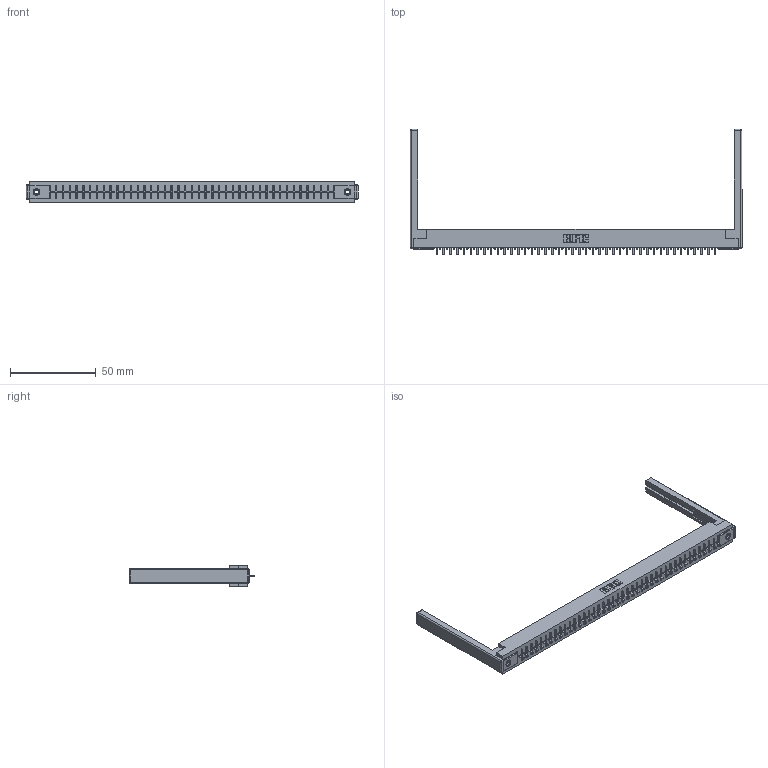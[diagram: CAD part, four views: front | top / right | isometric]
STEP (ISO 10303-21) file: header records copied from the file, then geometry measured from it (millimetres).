
FILE_DESCRIPTION (( 'STEP AP203' ), '1' );
FILE_NAME ('306-042-521-168.STEP', '2019-09-12T00:56:24', ( '' ), ( '' ), 'SwSTEP 2.0', 'SolidWorks 2016', '' );
FILE_SCHEMA (( 'CONFIG_CONTROL_DESIGN' ));
Length unit declared in the file: inch
Products named in the file (5): 345-250-001_345-250-001-102; 306-042-521-168; 307-220-068; 306-290-001_121; 306 Part_.156 Dia
Assembly tree (47 placements, depth 2):
  306-042-521-168
    306 Part_.156 Dia
    306-290-001_121  x42
    345-250-001_345-250-001-102  x2
    307-220-068  x2
Bounding box: 193.85 x 73.18 x 12.7 mm (x, y, z)
Volume: 25746 mm3; surface area: 25704.6 mm2
Topology: 47 solids, 47 shells, 3210 faces, 8980 edges, 5740 vertices
Faces by surface type: plane 2130, cylinder 888, sphere 176, cone 12, torus 4
Entity records: 41882 total; most frequent: CARTESIAN_POINT 6998, ORIENTED_EDGE 6930, DIRECTION 6913, EDGE_CURVE 3465, VECTOR 2707, LINE 2707, VERTEX_POINT 2188, AXIS2_PLACEMENT_3D 2103
